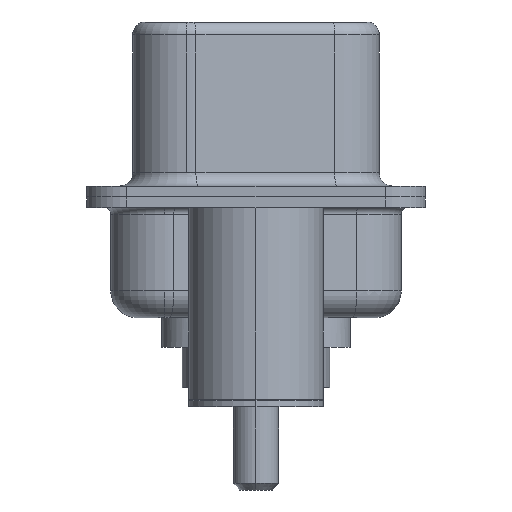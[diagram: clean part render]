
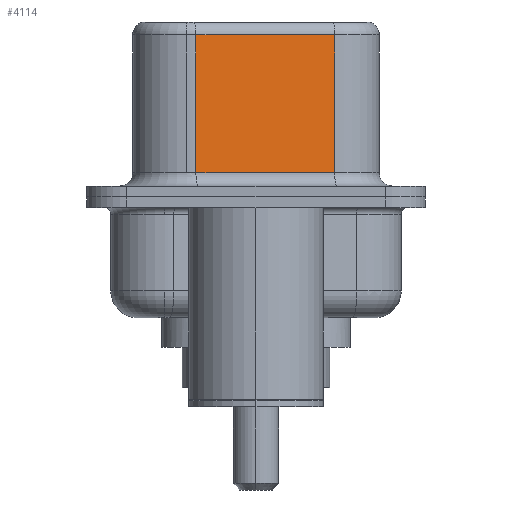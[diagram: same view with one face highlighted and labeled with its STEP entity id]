
A CAD part, left-side view. The second image highlights one B-rep face of the part: STEP entity #4114.
In plain terms, the highlighted planar face has unit normal (-0.985, -0.174, 0).
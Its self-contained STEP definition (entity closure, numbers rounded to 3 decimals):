
#475 = VECTOR ( 'NONE', #11669, 1000. ) ;
#703 = ORIENTED_EDGE ( 'NONE', *, *, #9807, .T. ) ;
#784 = LINE ( 'NONE', #12570, #475 ) ;
#820 = ORIENTED_EDGE ( 'NONE', *, *, #9711, .F. ) ;
#1875 = VECTOR ( 'NONE', #3121, 1000. ) ;
#1911 = CARTESIAN_POINT ( 'NONE',  ( 4.565, -2.927, 6.52 ) ) ;
#2145 = CARTESIAN_POINT ( 'NONE',  ( 4.565, -2.927, 6.52 ) ) ;
#2264 = CARTESIAN_POINT ( 'NONE',  ( 4.565, -2.927, 6.02 ) ) ;
#2803 = VERTEX_POINT ( 'NONE', #9379 ) ;
#2889 = ORIENTED_EDGE ( 'NONE', *, *, #8934, .T. ) ;
#2900 = DIRECTION ( 'NONE',  ( 0., 0., -1. ) ) ;
#3121 = DIRECTION ( 'NONE',  ( -0.174, 0.985, 0. ) ) ;
#4114 = ADVANCED_FACE ( 'NONE', ( #8507 ), #5888, .F. ) ;
#4227 = ORIENTED_EDGE ( 'NONE', *, *, #4795, .T. ) ;
#4795 = EDGE_CURVE ( 'NONE', #6189, #10440, #784, .T. ) ;
#5037 = CARTESIAN_POINT ( 'NONE',  ( 3.655, 2.233, 0.9 ) ) ;
#5141 = CARTESIAN_POINT ( 'NONE',  ( 4.565, -2.927, 0.9 ) ) ;
#5736 = DIRECTION ( 'NONE',  ( -0.174, 0.985, 0. ) ) ;
#5779 = DIRECTION ( 'NONE',  ( 0.985, 0.174, 0. ) ) ;
#5888 = PLANE ( 'NONE',  #12361 ) ;
#6189 = VERTEX_POINT ( 'NONE', #9576 ) ;
#6881 = EDGE_LOOP ( 'NONE', ( #820, #2889, #4227, #703 ) ) ;
#7463 = LINE ( 'NONE', #2264, #1875 ) ;
#7773 = VECTOR ( 'NONE', #2900, 1000. ) ;
#8507 = FACE_OUTER_BOUND ( 'NONE', #6881, .T. ) ;
#8934 = EDGE_CURVE ( 'NONE', #2803, #6189, #7463, .T. ) ;
#9254 = VECTOR ( 'NONE', #12495, 1000. ) ;
#9266 = VERTEX_POINT ( 'NONE', #10500 ) ;
#9379 = CARTESIAN_POINT ( 'NONE',  ( 4.565, -2.927, 6.02 ) ) ;
#9576 = CARTESIAN_POINT ( 'NONE',  ( 3.655, 2.233, 6.02 ) ) ;
#9711 = EDGE_CURVE ( 'NONE', #2803, #9266, #13279, .T. ) ;
#9807 = EDGE_CURVE ( 'NONE', #10440, #9266, #11975, .T. ) ;
#10440 = VERTEX_POINT ( 'NONE', #5037 ) ;
#10500 = CARTESIAN_POINT ( 'NONE',  ( 4.565, -2.927, 0.9 ) ) ;
#11669 = DIRECTION ( 'NONE',  ( 0., 0., -1. ) ) ;
#11975 = LINE ( 'NONE', #5141, #9254 ) ;
#12361 = AXIS2_PLACEMENT_3D ( 'NONE', #2145, #5779, #5736 ) ;
#12495 = DIRECTION ( 'NONE',  ( 0.174, -0.985, 0. ) ) ;
#12570 = CARTESIAN_POINT ( 'NONE',  ( 3.655, 2.233, 6.52 ) ) ;
#13279 = LINE ( 'NONE', #1911, #7773 ) ;
